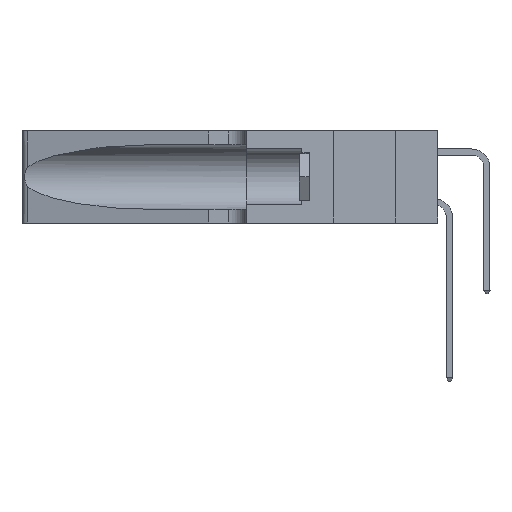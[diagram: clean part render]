
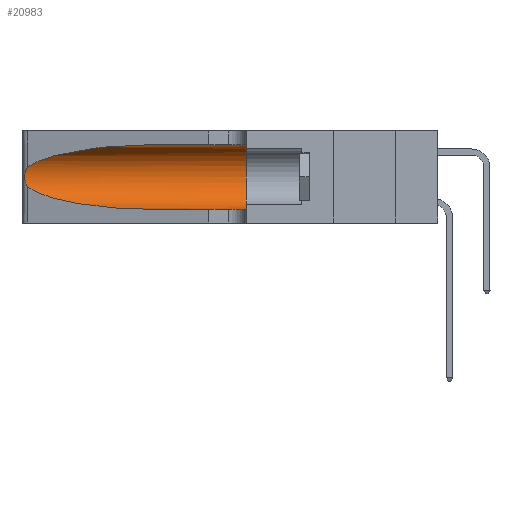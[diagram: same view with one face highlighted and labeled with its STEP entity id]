
A CAD part, left-side view. The second image highlights one B-rep face of the part: STEP entity #20983.
In plain terms, the highlighted cylindrical face has radius 3.308 mm (diameter 6.617 mm), a partial arc.
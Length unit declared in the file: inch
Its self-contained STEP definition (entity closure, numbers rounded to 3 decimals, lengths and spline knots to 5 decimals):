
#131 = ORIENTED_EDGE ( 'NONE', *, *, #3586, .T. ) ;
#871 = VECTOR ( 'NONE', #41585, 39.37008 ) ;
#1810 = CARTESIAN_POINT ( 'NONE',  ( 0.25487, 1.22718, 0.22369 ) ) ;
#2211 = VECTOR ( 'NONE', #29713, 39.37008 ) ;
#2943 = CARTESIAN_POINT ( 'NONE',  ( 0.1305, 0.35, 0.185 ) ) ;
#3005 = LINE ( 'NONE', #22027, #871 ) ;
#3292 = AXIS2_PLACEMENT_3D ( 'NONE', #28248, #38113, #21696 ) ;
#3341 = ORIENTED_EDGE ( 'NONE', *, *, #23390, .F. ) ;
#3372 = CARTESIAN_POINT ( 'NONE',  ( 0.25856, 1.23593, 0.16098 ) ) ;
#3586 = EDGE_CURVE ( 'NONE', #26482, #17811, #3838, .T. ) ;
#3760 = CARTESIAN_POINT ( 'NONE',  ( 0.18966, 0.96281, 0.05475 ) ) ;
#3838 = B_SPLINE_CURVE_WITH_KNOTS ( 'NONE', 3,
 ( #13337, #32979, #29706, #36301, #16667, #39577, #20005, #19846, #23287, #3372, #26561, #6790, #29851, #10166 ),
 .UNSPECIFIED., .F., .F.,
 ( 4, 2, 2, 2, 2, 2, 4 ),
 ( 0., 0.00027, 0.00053, 0.00107, 0.0016, 0.00187, 0.00214 ),
 .UNSPECIFIED. ) ;
#6365 = DIRECTION ( 'NONE',  ( 0., 0., 1. ) ) ;
#6646 = CARTESIAN_POINT ( 'NONE',  ( 0.1305, 1.61858, 0.05475 ) ) ;
#6790 = CARTESIAN_POINT ( 'NONE',  ( 0.25639, 1.23186, 0.15144 ) ) ;
#7905 = AXIS2_PLACEMENT_3D ( 'NONE', #2943, #26151, #6365 ) ;
#10166 = CARTESIAN_POINT ( 'NONE',  ( 0.25487, 1.22718, 0.14631 ) ) ;
#10463 = CARTESIAN_POINT ( 'NONE',  ( 0.1305, 0.35, 0.31525 ) ) ;
#12516 = EDGE_CURVE ( 'NONE', #17811, #37343, #16138, .T. ) ;
#13213 = CARTESIAN_POINT ( 'NONE',  ( 0.1305, 0.72297, 0.31525 ) ) ;
#13337 = CARTESIAN_POINT ( 'NONE',  ( 0.25487, 1.22718, 0.22369 ) ) ;
#14010 = CYLINDRICAL_SURFACE ( 'NONE', #3292, 0.13025 ) ;
#15041 = FACE_OUTER_BOUND ( 'NONE', #41839, .T. ) ;
#16138 =( BOUNDED_CURVE ( )  B_SPLINE_CURVE ( 3, ( #17042, #20361, #3760, #26913 ),
 .UNSPECIFIED., .F., .F. ) 
 B_SPLINE_CURVE_WITH_KNOTS ( ( 4, 4 ),
 ( 3.44316, 4.71239 ),
 .UNSPECIFIED. ) 
 CURVE ( )  GEOMETRIC_REPRESENTATION_ITEM ( )  RATIONAL_B_SPLINE_CURVE ( ( 1., 0.87, 0.87, 1. ) ) 
 REPRESENTATION_ITEM ( '' )  );
#16667 = CARTESIAN_POINT ( 'NONE',  ( 0.25854, 1.2359, 0.20912 ) ) ;
#17042 = CARTESIAN_POINT ( 'NONE',  ( 0.25487, 1.22718, 0.14631 ) ) ;
#17310 = CARTESIAN_POINT ( 'NONE',  ( 0.1305, 0.72297, 0.05475 ) ) ;
#17811 = VERTEX_POINT ( 'NONE', #24553 ) ;
#17988 = ORIENTED_EDGE ( 'NONE', *, *, #12516, .T. ) ;
#19846 = CARTESIAN_POINT ( 'NONE',  ( 0.26075, 1.23896, 0.178 ) ) ;
#20005 = CARTESIAN_POINT ( 'NONE',  ( 0.26075, 1.23896, 0.19203 ) ) ;
#20361 = CARTESIAN_POINT ( 'NONE',  ( 0.2373, 1.15595, 0.08982 ) ) ;
#20983 = ADVANCED_FACE ( 'NONE', ( #15041 ), #14010, .F. ) ;
#21062 = ORIENTED_EDGE ( 'NONE', *, *, #40344, .F. ) ;
#21696 = DIRECTION ( 'NONE',  ( 0., 0., -1. ) ) ;
#21811 = CARTESIAN_POINT ( 'NONE',  ( 0.2373, 1.15595, 0.28018 ) ) ;
#22027 = CARTESIAN_POINT ( 'NONE',  ( 0.1305, 1.61858, 0.31525 ) ) ;
#23287 = CARTESIAN_POINT ( 'NONE',  ( 0.26017, 1.23833, 0.17102 ) ) ;
#23390 = EDGE_CURVE ( 'NONE', #23543, #33753, #34887, .T. ) ;
#23441 = VERTEX_POINT ( 'NONE', #13213 ) ;
#23543 = VERTEX_POINT ( 'NONE', #10463 ) ;
#24553 = CARTESIAN_POINT ( 'NONE',  ( 0.25487, 1.22718, 0.14631 ) ) ;
#26151 = DIRECTION ( 'NONE',  ( 0., 1., 0. ) ) ;
#26482 = VERTEX_POINT ( 'NONE', #28693 ) ;
#26561 = CARTESIAN_POINT ( 'NONE',  ( 0.25789, 1.23486, 0.15765 ) ) ;
#26666 = ORIENTED_EDGE ( 'NONE', *, *, #29370, .T. ) ;
#26913 = CARTESIAN_POINT ( 'NONE',  ( 0.1305, 0.72297, 0.05475 ) ) ;
#28248 = CARTESIAN_POINT ( 'NONE',  ( 0.1305, 1.61858, 0.185 ) ) ;
#28669 = LINE ( 'NONE', #6646, #2211 ) ;
#28693 = CARTESIAN_POINT ( 'NONE',  ( 0.25487, 1.22718, 0.22369 ) ) ;
#29370 = EDGE_CURVE ( 'NONE', #37343, #33753, #28669, .T. ) ;
#29706 = CARTESIAN_POINT ( 'NONE',  ( 0.25639, 1.23184, 0.21858 ) ) ;
#29713 = DIRECTION ( 'NONE',  ( 0., -1., 0. ) ) ;
#29851 = CARTESIAN_POINT ( 'NONE',  ( 0.25555, 1.22993, 0.14849 ) ) ;
#30377 = EDGE_CURVE ( 'NONE', #23441, #26482, #32675, .T. ) ;
#31271 = ORIENTED_EDGE ( 'NONE', *, *, #30377, .T. ) ;
#32675 =( BOUNDED_CURVE ( )  B_SPLINE_CURVE ( 3, ( #37948, #34809, #21811, #1810 ),
 .UNSPECIFIED., .F., .F. ) 
 B_SPLINE_CURVE_WITH_KNOTS ( ( 4, 4 ),
 ( 1.5708, 2.84003 ),
 .UNSPECIFIED. ) 
 CURVE ( )  GEOMETRIC_REPRESENTATION_ITEM ( )  RATIONAL_B_SPLINE_CURVE ( ( 1., 0.87, 0.87, 1. ) ) 
 REPRESENTATION_ITEM ( '' )  );
#32979 = CARTESIAN_POINT ( 'NONE',  ( 0.25555, 1.22994, 0.2215 ) ) ;
#33753 = VERTEX_POINT ( 'NONE', #42382 ) ;
#34809 = CARTESIAN_POINT ( 'NONE',  ( 0.18966, 0.96281, 0.31525 ) ) ;
#34887 = CIRCLE ( 'NONE', #7905, 0.13025 ) ;
#36301 = CARTESIAN_POINT ( 'NONE',  ( 0.25787, 1.23484, 0.2124 ) ) ;
#37343 = VERTEX_POINT ( 'NONE', #17310 ) ;
#37948 = CARTESIAN_POINT ( 'NONE',  ( 0.1305, 0.72297, 0.31525 ) ) ;
#38113 = DIRECTION ( 'NONE',  ( 0., -1., 0. ) ) ;
#39577 = CARTESIAN_POINT ( 'NONE',  ( 0.26018, 1.23835, 0.19895 ) ) ;
#40344 = EDGE_CURVE ( 'NONE', #23441, #23543, #3005, .T. ) ;
#41585 = DIRECTION ( 'NONE',  ( 0., -1., 0. ) ) ;
#41839 = EDGE_LOOP ( 'NONE', ( #31271, #131, #17988, #26666, #3341, #21062 ) ) ;
#42382 = CARTESIAN_POINT ( 'NONE',  ( 0.1305, 0.35, 0.05475 ) ) ;
